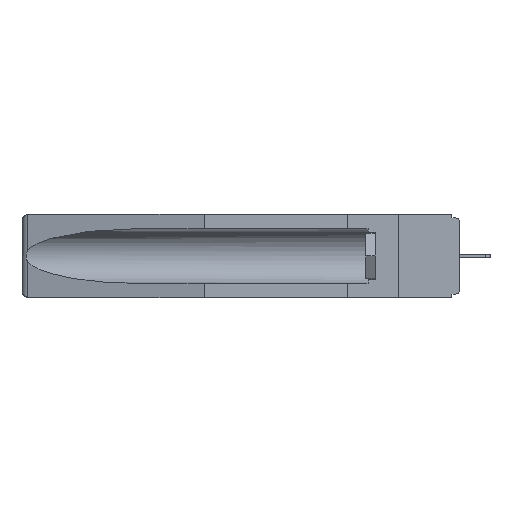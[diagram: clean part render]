
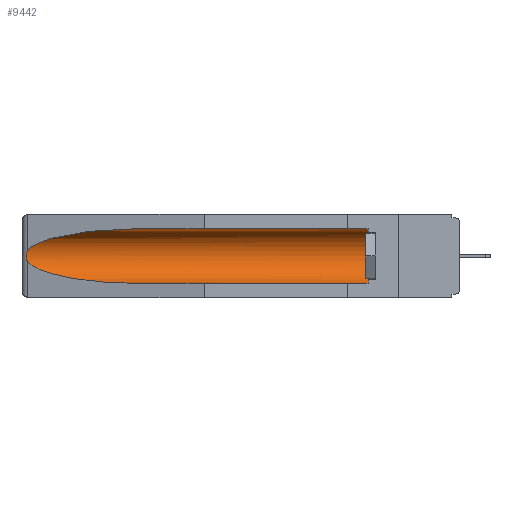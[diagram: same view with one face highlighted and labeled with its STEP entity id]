
A CAD part, left-side view. The second image highlights one B-rep face of the part: STEP entity #9442.
In plain terms, the highlighted cylindrical face has radius 2.857 mm (diameter 5.715 mm), a partial arc.
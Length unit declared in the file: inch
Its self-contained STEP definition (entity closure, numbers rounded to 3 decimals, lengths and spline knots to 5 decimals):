
#563 = ORIENTED_EDGE ( 'NONE', *, *, #19946, .T. ) ;
#818 = CARTESIAN_POINT ( 'NONE',  ( 0.155, 1.07973, -0.059 ) ) ;
#950 = VERTEX_POINT ( 'NONE', #20819 ) ;
#1129 = VERTEX_POINT ( 'NONE', #16179 ) ;
#1406 = CARTESIAN_POINT ( 'NONE',  ( 0.155, 1.07973, -0.284 ) ) ;
#1803 = EDGE_CURVE ( 'NONE', #7826, #950, #8428, .T. ) ;
#2392 = VECTOR ( 'NONE', #8674, 39.37008 ) ;
#2526 = CARTESIAN_POINT ( 'NONE',  ( 0.25451, 1.48313, -0.09465 ) ) ;
#2964 =( BOUNDED_CURVE ( )  B_SPLINE_CURVE ( 3, ( #5577, #7299, #18755, #8998 ),
 .UNSPECIFIED., .F., .F. ) 
 B_SPLINE_CURVE_WITH_KNOTS ( ( 4, 4 ),
 ( 0.1948, 1.5708 ),
 .UNSPECIFIED. ) 
 CURVE ( )  GEOMETRIC_REPRESENTATION_ITEM ( )  RATIONAL_B_SPLINE_CURVE ( ( 1., 0.848, 0.848, 1. ) ) 
 REPRESENTATION_ITEM ( '' )  );
#3076 = FACE_OUTER_BOUND ( 'NONE', #20213, .T. ) ;
#3720 = CARTESIAN_POINT ( 'NONE',  ( 0.155, -0.30754, -0.1715 ) ) ;
#3753 = CARTESIAN_POINT ( 'NONE',  ( 0.155, 0.126, -0.284 ) ) ;
#4111 = AXIS2_PLACEMENT_3D ( 'NONE', #3720, #10402, #15301 ) ;
#4112 = CARTESIAN_POINT ( 'NONE',  ( 0.2673, 1.5327, -0.16383 ) ) ;
#4333 = B_SPLINE_CURVE_WITH_KNOTS ( 'NONE', 3,
 ( #5762, #9156, #14032, #4112, #15672, #5828, #17314, #7565, #19015, #9229 ),
 .UNSPECIFIED., .F., .F.,
 ( 4, 2, 2, 2, 4 ),
 ( 0., 0.00029, 0.00058, 0.00087, 0.00117 ),
 .UNSPECIFIED. ) ;
#4578 =( BOUNDED_CURVE ( )  B_SPLINE_CURVE ( 3, ( #818, #12509, #2526, #14134 ),
 .UNSPECIFIED., .F., .T. ) 
 B_SPLINE_CURVE_WITH_KNOTS ( ( 4, 4 ),
 ( 4.71239, 6.08839 ),
 .UNSPECIFIED. ) 
 CURVE ( )  GEOMETRIC_REPRESENTATION_ITEM ( )  RATIONAL_B_SPLINE_CURVE ( ( 1., 0.848, 0.848, 1. ) ) 
 REPRESENTATION_ITEM ( '' )  );
#4983 = VERTEX_POINT ( 'NONE', #3753 ) ;
#5577 = CARTESIAN_POINT ( 'NONE',  ( 0.26537, 1.52718, -0.19328 ) ) ;
#5762 = CARTESIAN_POINT ( 'NONE',  ( 0.26537, 1.52718, -0.14972 ) ) ;
#5828 = CARTESIAN_POINT ( 'NONE',  ( 0.2675, 1.53308, -0.17534 ) ) ;
#6221 = CIRCLE ( 'NONE', #21017, 0.1125 ) ;
#6472 = VERTEX_POINT ( 'NONE', #1406 ) ;
#6908 = LINE ( 'NONE', #20110, #2392 ) ;
#7299 = CARTESIAN_POINT ( 'NONE',  ( 0.25451, 1.48313, -0.24835 ) ) ;
#7328 = ORIENTED_EDGE ( 'NONE', *, *, #1803, .T. ) ;
#7565 = CARTESIAN_POINT ( 'NONE',  ( 0.26655, 1.53094, -0.18657 ) ) ;
#7715 = EDGE_CURVE ( 'NONE', #12430, #6472, #2964, .T. ) ;
#7826 = VERTEX_POINT ( 'NONE', #10816 ) ;
#7903 = VECTOR ( 'NONE', #15175, 39.37008 ) ;
#8057 = ORIENTED_EDGE ( 'NONE', *, *, #16514, .T. ) ;
#8335 = DIRECTION ( 'NONE',  ( 0., -1., 0. ) ) ;
#8428 = LINE ( 'NONE', #14749, #7903 ) ;
#8674 = DIRECTION ( 'NONE',  ( 0., 1., 0. ) ) ;
#8998 = CARTESIAN_POINT ( 'NONE',  ( 0.155, 1.07973, -0.284 ) ) ;
#9156 = CARTESIAN_POINT ( 'NONE',  ( 0.26597, 1.52961, -0.15275 ) ) ;
#9229 = CARTESIAN_POINT ( 'NONE',  ( 0.26537, 1.52718, -0.19328 ) ) ;
#9442 = ADVANCED_FACE ( 'NONE', ( #3076 ), #11416, .F. ) ;
#9637 = ORIENTED_EDGE ( 'NONE', *, *, #10216, .T. ) ;
#10216 = EDGE_CURVE ( 'NONE', #4983, #7826, #6221, .T. ) ;
#10402 = DIRECTION ( 'NONE',  ( 0., 1., 0. ) ) ;
#10523 = ORIENTED_EDGE ( 'NONE', *, *, #12737, .F. ) ;
#10816 = CARTESIAN_POINT ( 'NONE',  ( 0.155, 0.126, -0.059 ) ) ;
#11416 = CYLINDRICAL_SURFACE ( 'NONE', #4111, 0.1125 ) ;
#12430 = VERTEX_POINT ( 'NONE', #13981 ) ;
#12509 = CARTESIAN_POINT ( 'NONE',  ( 0.21114, 1.30732, -0.059 ) ) ;
#12737 = EDGE_CURVE ( 'NONE', #4983, #6472, #6908, .T. ) ;
#13981 = CARTESIAN_POINT ( 'NONE',  ( 0.26537, 1.52718, -0.19328 ) ) ;
#14032 = CARTESIAN_POINT ( 'NONE',  ( 0.26654, 1.53092, -0.15636 ) ) ;
#14134 = CARTESIAN_POINT ( 'NONE',  ( 0.26537, 1.52718, -0.14972 ) ) ;
#14749 = CARTESIAN_POINT ( 'NONE',  ( 0.155, -0.30754, -0.059 ) ) ;
#15175 = DIRECTION ( 'NONE',  ( 0., 1., 0. ) ) ;
#15301 = DIRECTION ( 'NONE',  ( 0., 0., 1. ) ) ;
#15672 = CARTESIAN_POINT ( 'NONE',  ( 0.2675, 1.53308, -0.16763 ) ) ;
#16179 = CARTESIAN_POINT ( 'NONE',  ( 0.26537, 1.52718, -0.14972 ) ) ;
#16514 = EDGE_CURVE ( 'NONE', #950, #1129, #4578, .T. ) ;
#17314 = CARTESIAN_POINT ( 'NONE',  ( 0.2673, 1.53269, -0.17917 ) ) ;
#18103 = CARTESIAN_POINT ( 'NONE',  ( 0.155, 0.126, -0.1715 ) ) ;
#18755 = CARTESIAN_POINT ( 'NONE',  ( 0.21114, 1.30732, -0.284 ) ) ;
#19015 = CARTESIAN_POINT ( 'NONE',  ( 0.26597, 1.5296, -0.19026 ) ) ;
#19780 = DIRECTION ( 'NONE',  ( 0., 0., 1. ) ) ;
#19946 = EDGE_CURVE ( 'NONE', #1129, #12430, #4333, .T. ) ;
#20110 = CARTESIAN_POINT ( 'NONE',  ( 0.155, -0.30754, -0.284 ) ) ;
#20213 = EDGE_LOOP ( 'NONE', ( #8057, #563, #20536, #10523, #9637, #7328 ) ) ;
#20536 = ORIENTED_EDGE ( 'NONE', *, *, #7715, .T. ) ;
#20819 = CARTESIAN_POINT ( 'NONE',  ( 0.155, 1.07973, -0.059 ) ) ;
#21017 = AXIS2_PLACEMENT_3D ( 'NONE', #18103, #8335, #19780 ) ;
